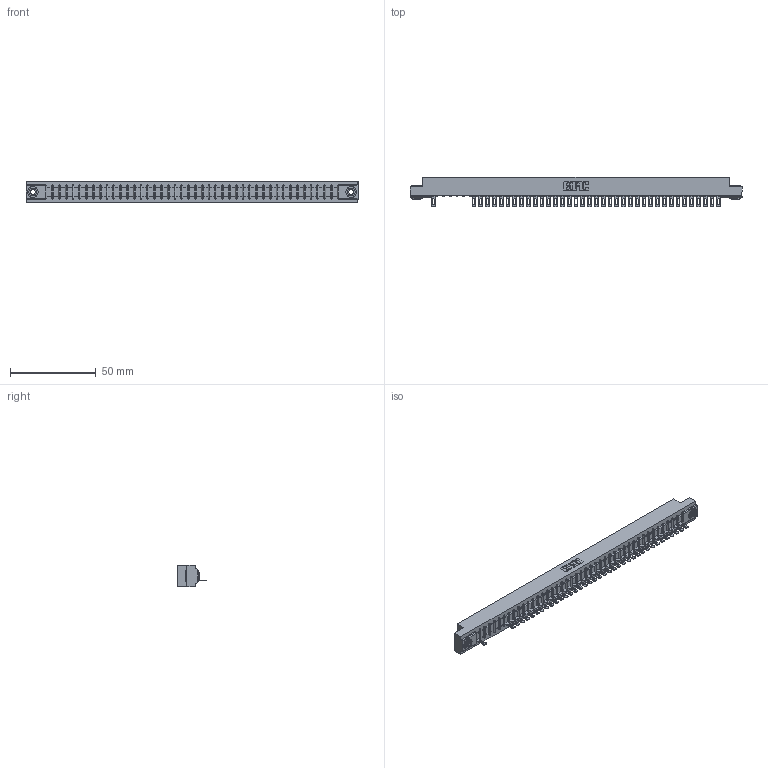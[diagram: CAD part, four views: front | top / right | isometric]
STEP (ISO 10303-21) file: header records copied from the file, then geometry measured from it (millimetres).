
FILE_DESCRIPTION (( 'STEP AP203' ), '1' );
FILE_NAME ('357-043-501-103.STEP', '2018-08-11T10:07:56', ( '' ), ( '' ), 'SwSTEP 2.0', 'SolidWorks 2016', '' );
FILE_SCHEMA (( 'CONFIG_CONTROL_DESIGN' ));
Length unit declared in the file: inch
Products named in the file (4): 345-250-002_345-250-002-102; 357-043-501-103; 307 Part_.156 Dia Mounting Holes; 307-290-002_501
Assembly tree (41 placements, depth 2):
  357-043-501-103
    307 Part_.156 Dia Mounting Holes
    307-290-002_501  x38
    345-250-002_345-250-002-102  x2
Bounding box: 193.4 x 17.42 x 12.7 mm (x, y, z)
Volume: 20592.9 mm3; surface area: 25493.7 mm2
Topology: 41 solids, 41 shells, 3202 faces, 9799 edges, 6410 vertices
Faces by surface type: plane 1826, cylinder 1280, sphere 88, cone 8
Entity records: 38439 total; most frequent: CARTESIAN_POINT 6484, ORIENTED_EDGE 6470, DIRECTION 6313, EDGE_CURVE 3235, LINE 2467, VECTOR 2467, VERTEX_POINT 2094, AXIS2_PLACEMENT_3D 1923
